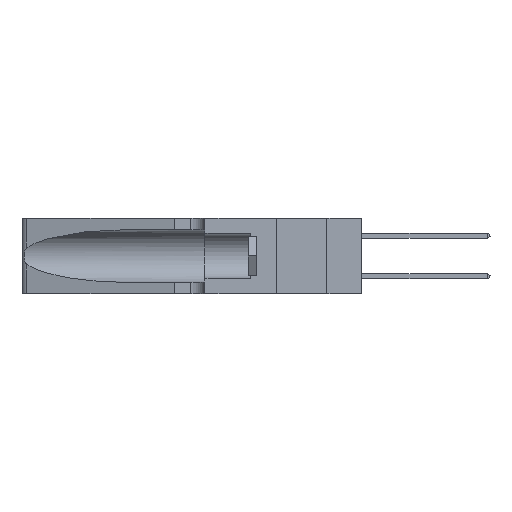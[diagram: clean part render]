
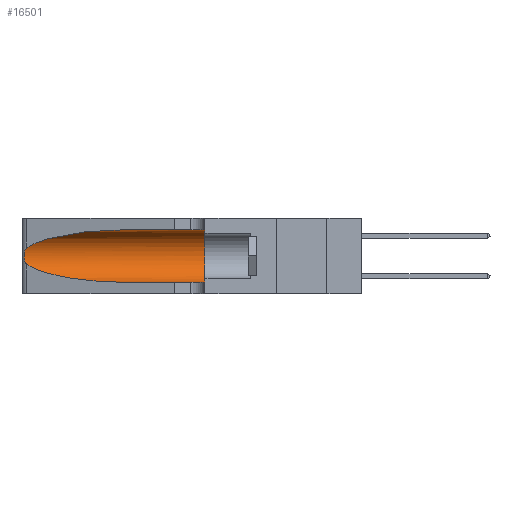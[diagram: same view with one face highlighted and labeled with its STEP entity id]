
A CAD part, left-side view. The second image highlights one B-rep face of the part: STEP entity #16501.
In plain terms, the highlighted cylindrical face has radius 3.308 mm (diameter 6.617 mm), a partial arc.
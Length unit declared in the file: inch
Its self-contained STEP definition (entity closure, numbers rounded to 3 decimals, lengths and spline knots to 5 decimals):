
#124 = VERTEX_POINT ( 'NONE', #35802 ) ;
#477 = FACE_OUTER_BOUND ( 'NONE', #24661, .T. ) ;
#1192 = CARTESIAN_POINT ( 'NONE',  ( 0.1305, 0.35, 0.185 ) ) ;
#1384 = VERTEX_POINT ( 'NONE', #42515 ) ;
#1832 = ORIENTED_EDGE ( 'NONE', *, *, #41274, .T. ) ;
#1938 = EDGE_CURVE ( 'NONE', #1384, #22424, #36596, .T. ) ;
#3123 = CARTESIAN_POINT ( 'NONE',  ( 0.26017, 1.23833, 0.17102 ) ) ;
#3370 = EDGE_CURVE ( 'NONE', #124, #38894, #28945, .T. ) ;
#6194 = CARTESIAN_POINT ( 'NONE',  ( 0.26075, 1.23896, 0.178 ) ) ;
#6485 = CARTESIAN_POINT ( 'NONE',  ( 0.25639, 1.23186, 0.15144 ) ) ;
#6636 = CARTESIAN_POINT ( 'NONE',  ( 0.25487, 1.22718, 0.14631 ) ) ;
#7495 = ORIENTED_EDGE ( 'NONE', *, *, #1938, .T. ) ;
#7620 = CARTESIAN_POINT ( 'NONE',  ( 0.2373, 1.15595, 0.08982 ) ) ;
#9185 = VECTOR ( 'NONE', #25538, 39.37008 ) ;
#9615 = ORIENTED_EDGE ( 'NONE', *, *, #20284, .T. ) ;
#9993 = CARTESIAN_POINT ( 'NONE',  ( 0.25555, 1.22994, 0.2215 ) ) ;
#12052 = VERTEX_POINT ( 'NONE', #29526 ) ;
#13133 = ORIENTED_EDGE ( 'NONE', *, *, #33709, .F. ) ;
#13219 = CARTESIAN_POINT ( 'NONE',  ( 0.25555, 1.22993, 0.14849 ) ) ;
#13947 = EDGE_CURVE ( 'NONE', #124, #1384, #30759, .T. ) ;
#16501 = ADVANCED_FACE ( 'NONE', ( #477 ), #25981, .F. ) ;
#19288 = AXIS2_PLACEMENT_3D ( 'NONE', #1192, #37580, #38281 ) ;
#19728 = CARTESIAN_POINT ( 'NONE',  ( 0.25639, 1.23184, 0.21858 ) ) ;
#20284 = EDGE_CURVE ( 'NONE', #22424, #12052, #25655, .T. ) ;
#20988 = DIRECTION ( 'NONE',  ( 0., 0., -1. ) ) ;
#21292 = CARTESIAN_POINT ( 'NONE',  ( 0.25487, 1.22718, 0.14631 ) ) ;
#21587 = CARTESIAN_POINT ( 'NONE',  ( 0.1305, 0.72297, 0.05475 ) ) ;
#22424 = VERTEX_POINT ( 'NONE', #33206 ) ;
#22810 = CARTESIAN_POINT ( 'NONE',  ( 0.1305, 1.61858, 0.05475 ) ) ;
#22918 = CARTESIAN_POINT ( 'NONE',  ( 0.25487, 1.22718, 0.22369 ) ) ;
#24038 = DIRECTION ( 'NONE',  ( 0., -1., 0. ) ) ;
#24661 = EDGE_LOOP ( 'NONE', ( #33016, #7495, #9615, #1832, #13133, #27515 ) ) ;
#25112 = VERTEX_POINT ( 'NONE', #42022 ) ;
#25331 = CARTESIAN_POINT ( 'NONE',  ( 0.2373, 1.15595, 0.28018 ) ) ;
#25538 = DIRECTION ( 'NONE',  ( 0., -1., 0. ) ) ;
#25594 = AXIS2_PLACEMENT_3D ( 'NONE', #26483, #24038, #20988 ) ;
#25655 =( BOUNDED_CURVE ( )  B_SPLINE_CURVE ( 3, ( #21292, #7620, #27666, #21587 ),
 .UNSPECIFIED., .F., .T. ) 
 B_SPLINE_CURVE_WITH_KNOTS ( ( 4, 4 ),
 ( 3.44316, 4.71239 ),
 .UNSPECIFIED. ) 
 CURVE ( )  GEOMETRIC_REPRESENTATION_ITEM ( )  RATIONAL_B_SPLINE_CURVE ( ( 1., 0.87, 0.87, 1. ) ) 
 REPRESENTATION_ITEM ( '' )  );
#25785 = VECTOR ( 'NONE', #28198, 39.37008 ) ;
#25814 = CARTESIAN_POINT ( 'NONE',  ( 0.1305, 1.61858, 0.31525 ) ) ;
#25981 = CYLINDRICAL_SURFACE ( 'NONE', #25594, 0.13025 ) ;
#26110 = CARTESIAN_POINT ( 'NONE',  ( 0.25787, 1.23484, 0.2124 ) ) ;
#26414 = CARTESIAN_POINT ( 'NONE',  ( 0.25789, 1.23486, 0.15765 ) ) ;
#26483 = CARTESIAN_POINT ( 'NONE',  ( 0.1305, 1.61858, 0.185 ) ) ;
#26556 = CARTESIAN_POINT ( 'NONE',  ( 0.25854, 1.2359, 0.20912 ) ) ;
#27515 = ORIENTED_EDGE ( 'NONE', *, *, #3370, .F. ) ;
#27666 = CARTESIAN_POINT ( 'NONE',  ( 0.18966, 0.96281, 0.05475 ) ) ;
#28198 = DIRECTION ( 'NONE',  ( 0., -1., 0. ) ) ;
#28945 = LINE ( 'NONE', #25814, #9185 ) ;
#29526 = CARTESIAN_POINT ( 'NONE',  ( 0.1305, 0.72297, 0.05475 ) ) ;
#29818 = CARTESIAN_POINT ( 'NONE',  ( 0.1305, 0.35, 0.31525 ) ) ;
#30759 =( BOUNDED_CURVE ( )  B_SPLINE_CURVE ( 3, ( #38529, #41604, #25331, #38795 ),
 .UNSPECIFIED., .F., .F. ) 
 B_SPLINE_CURVE_WITH_KNOTS ( ( 4, 4 ),
 ( 1.5708, 2.84003 ),
 .UNSPECIFIED. ) 
 CURVE ( )  GEOMETRIC_REPRESENTATION_ITEM ( )  RATIONAL_B_SPLINE_CURVE ( ( 1., 0.87, 0.87, 1. ) ) 
 REPRESENTATION_ITEM ( '' )  );
#33016 = ORIENTED_EDGE ( 'NONE', *, *, #13947, .T. ) ;
#33100 = CARTESIAN_POINT ( 'NONE',  ( 0.26075, 1.23896, 0.19203 ) ) ;
#33206 = CARTESIAN_POINT ( 'NONE',  ( 0.25487, 1.22718, 0.14631 ) ) ;
#33709 = EDGE_CURVE ( 'NONE', #38894, #25112, #39354, .T. ) ;
#34649 = LINE ( 'NONE', #22810, #25785 ) ;
#35802 = CARTESIAN_POINT ( 'NONE',  ( 0.1305, 0.72297, 0.31525 ) ) ;
#36439 = CARTESIAN_POINT ( 'NONE',  ( 0.25856, 1.23593, 0.16098 ) ) ;
#36587 = CARTESIAN_POINT ( 'NONE',  ( 0.26018, 1.23835, 0.19895 ) ) ;
#36596 = B_SPLINE_CURVE_WITH_KNOTS ( 'NONE', 3,
 ( #22918, #9993, #19728, #26110, #26556, #36587, #33100, #6194, #3123, #36439, #26414, #6485, #13219, #6636 ),
 .UNSPECIFIED., .F., .F.,
 ( 4, 2, 2, 2, 2, 2, 4 ),
 ( 0., 0.00027, 0.00053, 0.00107, 0.0016, 0.00187, 0.00214 ),
 .UNSPECIFIED. ) ;
#37580 = DIRECTION ( 'NONE',  ( 0., 1., 0. ) ) ;
#38281 = DIRECTION ( 'NONE',  ( 0., 0., 1. ) ) ;
#38529 = CARTESIAN_POINT ( 'NONE',  ( 0.1305, 0.72297, 0.31525 ) ) ;
#38795 = CARTESIAN_POINT ( 'NONE',  ( 0.25487, 1.22718, 0.22369 ) ) ;
#38894 = VERTEX_POINT ( 'NONE', #29818 ) ;
#39354 = CIRCLE ( 'NONE', #19288, 0.13025 ) ;
#41274 = EDGE_CURVE ( 'NONE', #12052, #25112, #34649, .T. ) ;
#41604 = CARTESIAN_POINT ( 'NONE',  ( 0.18966, 0.96281, 0.31525 ) ) ;
#42022 = CARTESIAN_POINT ( 'NONE',  ( 0.1305, 0.35, 0.05475 ) ) ;
#42515 = CARTESIAN_POINT ( 'NONE',  ( 0.25487, 1.22718, 0.22369 ) ) ;
